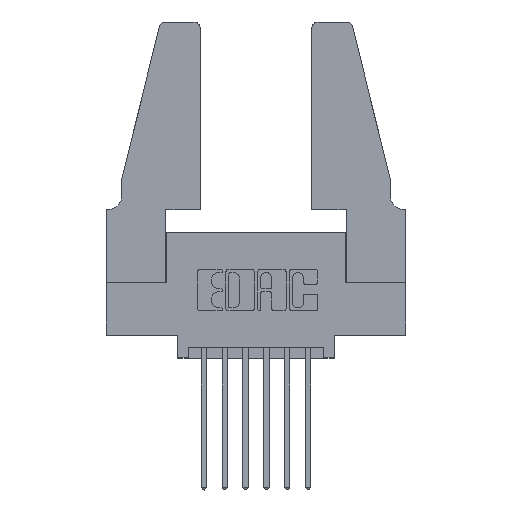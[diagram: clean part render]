
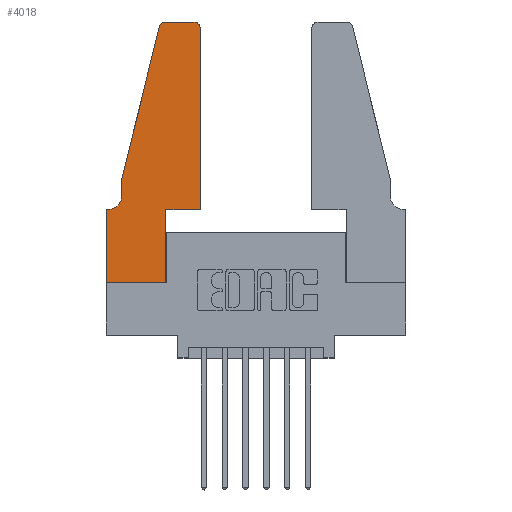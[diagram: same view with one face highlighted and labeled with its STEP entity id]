
A CAD part, top view. The second image highlights one B-rep face of the part: STEP entity #4018.
In plain terms, the highlighted planar face has unit normal (0, 0, 1).
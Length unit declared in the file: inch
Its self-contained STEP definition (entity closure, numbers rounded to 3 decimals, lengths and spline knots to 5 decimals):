
#87 = ORIENTED_EDGE ( 'NONE', *, *, #9015, .T. ) ;
#202 = LINE ( 'NONE', #7957, #9676 ) ;
#230 = CARTESIAN_POINT ( 'NONE',  ( 0.2865, 0.35, 0.37 ) ) ;
#339 = VERTEX_POINT ( 'NONE', #2315 ) ;
#363 = CARTESIAN_POINT ( 'NONE',  ( 0.0755, 0.5, 0.37 ) ) ;
#531 = AXIS2_PLACEMENT_3D ( 'NONE', #11431, #4823, #3982 ) ;
#916 = VERTEX_POINT ( 'NONE', #5775 ) ;
#1116 = EDGE_CURVE ( 'NONE', #1786, #4865, #10338, .T. ) ;
#1117 = VECTOR ( 'NONE', #4974, 39.37008 ) ;
#1388 = LINE ( 'NONE', #11669, #5408 ) ;
#1468 = EDGE_CURVE ( 'NONE', #2669, #1786, #7491, .T. ) ;
#1565 = LINE ( 'NONE', #2242, #1117 ) ;
#1639 = EDGE_CURVE ( 'NONE', #10920, #6350, #9355, .T. ) ;
#1747 = CARTESIAN_POINT ( 'NONE',  ( 0.4505, 1.22, 0.37 ) ) ;
#1786 = VERTEX_POINT ( 'NONE', #9506 ) ;
#1862 = CARTESIAN_POINT ( 'NONE',  ( 0.4205, 1.25, 0.37 ) ) ;
#2055 = DIRECTION ( 'NONE',  ( -1., 0., 0. ) ) ;
#2129 = CARTESIAN_POINT ( 'NONE',  ( 0.0055, 0.42, 0.37 ) ) ;
#2226 = ORIENTED_EDGE ( 'NONE', *, *, #1116, .T. ) ;
#2242 = CARTESIAN_POINT ( 'NONE',  ( 0.4505, 0.35, 0.37 ) ) ;
#2261 = DIRECTION ( 'NONE',  ( 0., 0., 1. ) ) ;
#2269 = CARTESIAN_POINT ( 'NONE',  ( 0.0755, 0.35, 0.37 ) ) ;
#2288 = ORIENTED_EDGE ( 'NONE', *, *, #9316, .T. ) ;
#2315 = CARTESIAN_POINT ( 'NONE',  ( 0., 0., 0.37 ) ) ;
#2414 = ORIENTED_EDGE ( 'NONE', *, *, #4546, .T. ) ;
#2425 = CARTESIAN_POINT ( 'NONE',  ( 0.0755, 0.5, 0.37 ) ) ;
#2429 = VERTEX_POINT ( 'NONE', #5745 ) ;
#2461 = VECTOR ( 'NONE', #8357, 39.37008 ) ;
#2539 = CARTESIAN_POINT ( 'NONE',  ( 0.0755, 0.42, 0.37 ) ) ;
#2669 = VERTEX_POINT ( 'NONE', #9596 ) ;
#2680 = DIRECTION ( 'NONE',  ( 1., 0., 0. ) ) ;
#2736 = AXIS2_PLACEMENT_3D ( 'NONE', #2129, #7522, #2055 ) ;
#2742 = CIRCLE ( 'NONE', #531, 0.03 ) ;
#2786 = EDGE_LOOP ( 'NONE', ( #4365, #8080, #2226, #87, #5330, #10209, #2288, #10460, #11854, #11269, #2414, #7876 ) ) ;
#3218 = EDGE_CURVE ( 'NONE', #6776, #7510, #2742, .T. ) ;
#3325 = DIRECTION ( 'NONE',  ( -1., 0., 0. ) ) ;
#3982 = DIRECTION ( 'NONE',  ( 1., 0., 0. ) ) ;
#4018 = ADVANCED_FACE ( 'NONE', ( #8727 ), #4043, .T. ) ;
#4043 = PLANE ( 'NONE',  #9059 ) ;
#4206 = LINE ( 'NONE', #11588, #10952 ) ;
#4309 = DIRECTION ( 'NONE',  ( 0., 1., 0. ) ) ;
#4365 = ORIENTED_EDGE ( 'NONE', *, *, #10703, .T. ) ;
#4546 = EDGE_CURVE ( 'NONE', #6350, #6776, #1565, .T. ) ;
#4773 = CARTESIAN_POINT ( 'NONE',  ( 0.0755, 0.5, 0.37 ) ) ;
#4823 = DIRECTION ( 'NONE',  ( 0., 0., 1. ) ) ;
#4854 = LINE ( 'NONE', #4773, #2461 ) ;
#4865 = VERTEX_POINT ( 'NONE', #2425 ) ;
#4974 = DIRECTION ( 'NONE',  ( 0., 1., 0. ) ) ;
#5112 = VERTEX_POINT ( 'NONE', #7600 ) ;
#5132 = CARTESIAN_POINT ( 'NONE',  ( 0.4505, 0.35, 0.37 ) ) ;
#5330 = ORIENTED_EDGE ( 'NONE', *, *, #11043, .T. ) ;
#5408 = VECTOR ( 'NONE', #6320, 39.37008 ) ;
#5473 = VECTOR ( 'NONE', #6018, 39.37008 ) ;
#5745 = CARTESIAN_POINT ( 'NONE',  ( 0., 0.35, 0.37 ) ) ;
#5775 = CARTESIAN_POINT ( 'NONE',  ( 0.0055, 0.35, 0.37 ) ) ;
#5829 = EDGE_CURVE ( 'NONE', #339, #5112, #7255, .T. ) ;
#6018 = DIRECTION ( 'NONE',  ( 1., 0., 0. ) ) ;
#6320 = DIRECTION ( 'NONE',  ( 0., -1., 0. ) ) ;
#6350 = VERTEX_POINT ( 'NONE', #5132 ) ;
#6776 = VERTEX_POINT ( 'NONE', #1747 ) ;
#6928 = CARTESIAN_POINT ( 'NONE',  ( 0.4505, 0.35, 0.37 ) ) ;
#7110 = EDGE_CURVE ( 'NONE', #5112, #10920, #4206, .T. ) ;
#7255 = LINE ( 'NONE', #9996, #10981 ) ;
#7420 = EDGE_CURVE ( 'NONE', #916, #2429, #10672, .T. ) ;
#7491 = CIRCLE ( 'NONE', #7618, 0.03 ) ;
#7510 = VERTEX_POINT ( 'NONE', #1862 ) ;
#7522 = DIRECTION ( 'NONE',  ( 0., 0., -1. ) ) ;
#7600 = CARTESIAN_POINT ( 'NONE',  ( 0.2865, 0., 0.37 ) ) ;
#7618 = AXIS2_PLACEMENT_3D ( 'NONE', #8110, #9940, #10787 ) ;
#7622 = VECTOR ( 'NONE', #3325, 39.37008 ) ;
#7626 = CIRCLE ( 'NONE', #2736, 0.07 ) ;
#7876 = ORIENTED_EDGE ( 'NONE', *, *, #3218, .T. ) ;
#7907 = VECTOR ( 'NONE', #10444, 39.37008 ) ;
#7957 = CARTESIAN_POINT ( 'NONE',  ( 0.2605, 1.25, 0.37 ) ) ;
#8080 = ORIENTED_EDGE ( 'NONE', *, *, #1468, .T. ) ;
#8110 = CARTESIAN_POINT ( 'NONE',  ( 0.284, 1.22, 0.37 ) ) ;
#8357 = DIRECTION ( 'NONE',  ( 0., -1., 0. ) ) ;
#8727 = FACE_OUTER_BOUND ( 'NONE', #2786, .T. ) ;
#9015 = EDGE_CURVE ( 'NONE', #4865, #11641, #4854, .T. ) ;
#9059 = AXIS2_PLACEMENT_3D ( 'NONE', #11298, #2261, #10355 ) ;
#9316 = EDGE_CURVE ( 'NONE', #2429, #339, #1388, .T. ) ;
#9355 = LINE ( 'NONE', #6928, #5473 ) ;
#9506 = CARTESIAN_POINT ( 'NONE',  ( 0.25487, 1.22718, 0.37 ) ) ;
#9596 = CARTESIAN_POINT ( 'NONE',  ( 0.284, 1.25, 0.37 ) ) ;
#9676 = VECTOR ( 'NONE', #10550, 39.37008 ) ;
#9940 = DIRECTION ( 'NONE',  ( 0., 0., 1. ) ) ;
#9996 = CARTESIAN_POINT ( 'NONE',  ( 0., 0., 0.37 ) ) ;
#10209 = ORIENTED_EDGE ( 'NONE', *, *, #7420, .T. ) ;
#10338 = LINE ( 'NONE', #363, #7907 ) ;
#10355 = DIRECTION ( 'NONE',  ( 1., 0., 0. ) ) ;
#10444 = DIRECTION ( 'NONE',  ( -0.239, -0.971, 0. ) ) ;
#10460 = ORIENTED_EDGE ( 'NONE', *, *, #5829, .T. ) ;
#10550 = DIRECTION ( 'NONE',  ( -1., 0., 0. ) ) ;
#10672 = LINE ( 'NONE', #2269, #7622 ) ;
#10703 = EDGE_CURVE ( 'NONE', #7510, #2669, #202, .T. ) ;
#10787 = DIRECTION ( 'NONE',  ( 1., 0., 0. ) ) ;
#10920 = VERTEX_POINT ( 'NONE', #230 ) ;
#10952 = VECTOR ( 'NONE', #4309, 39.37008 ) ;
#10981 = VECTOR ( 'NONE', #2680, 39.37008 ) ;
#11043 = EDGE_CURVE ( 'NONE', #11641, #916, #7626, .T. ) ;
#11269 = ORIENTED_EDGE ( 'NONE', *, *, #1639, .T. ) ;
#11298 = CARTESIAN_POINT ( 'NONE',  ( 0., 0.35, 0.37 ) ) ;
#11431 = CARTESIAN_POINT ( 'NONE',  ( 0.4205, 1.22, 0.37 ) ) ;
#11588 = CARTESIAN_POINT ( 'NONE',  ( 0.2865, 0.35, 0.37 ) ) ;
#11641 = VERTEX_POINT ( 'NONE', #2539 ) ;
#11669 = CARTESIAN_POINT ( 'NONE',  ( 0., 0., 0.37 ) ) ;
#11854 = ORIENTED_EDGE ( 'NONE', *, *, #7110, .T. ) ;
